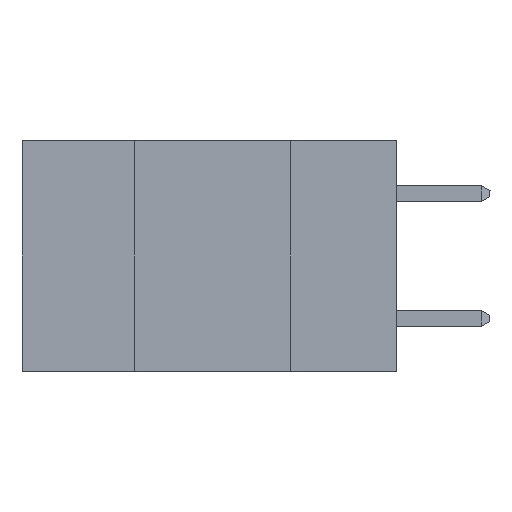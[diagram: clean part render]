
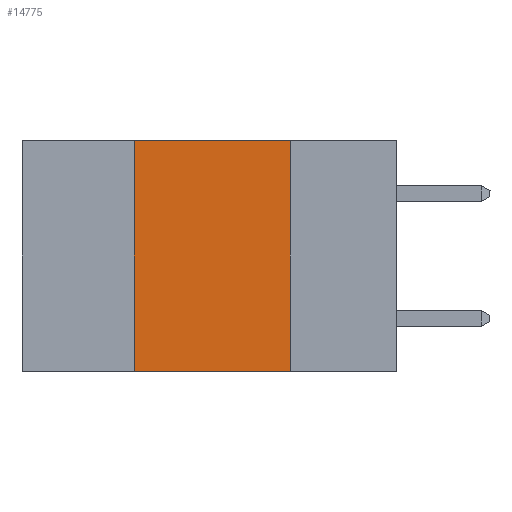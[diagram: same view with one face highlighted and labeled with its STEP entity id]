
A CAD part, left-side view. The second image highlights one B-rep face of the part: STEP entity #14775.
In plain terms, the highlighted planar face has unit normal (-1, 0, 0).
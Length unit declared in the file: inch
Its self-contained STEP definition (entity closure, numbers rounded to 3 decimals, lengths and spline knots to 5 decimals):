
#66 = CARTESIAN_POINT ( 'NONE',  ( 0., 0.42, 0. ) ) ;
#1553 = EDGE_CURVE ( 'NONE', #14657, #10902, #3819, .T. ) ;
#2326 = DIRECTION ( 'NONE',  ( 0., 0., 1. ) ) ;
#2853 = CARTESIAN_POINT ( 'NONE',  ( 0., 0.17, 0. ) ) ;
#3294 = CARTESIAN_POINT ( 'NONE',  ( 0., 0.17, 0. ) ) ;
#3672 = EDGE_CURVE ( 'NONE', #7648, #10902, #11378, .T. ) ;
#3819 = LINE ( 'NONE', #3294, #26152 ) ;
#4571 = VECTOR ( 'NONE', #2326, 39.37008 ) ;
#6388 = EDGE_LOOP ( 'NONE', ( #7945, #23681, #28286, #14852 ) ) ;
#6788 = DIRECTION ( 'NONE',  ( 0., 0., -1. ) ) ;
#6940 = FACE_OUTER_BOUND ( 'NONE', #6388, .T. ) ;
#7648 = VERTEX_POINT ( 'NONE', #14026 ) ;
#7729 = PLANE ( 'NONE',  #8079 ) ;
#7945 = ORIENTED_EDGE ( 'NONE', *, *, #1553, .F. ) ;
#8079 = AXIS2_PLACEMENT_3D ( 'NONE', #14413, #12248, #27793 ) ;
#8176 = EDGE_CURVE ( 'NONE', #7648, #18241, #10521, .T. ) ;
#9733 = CARTESIAN_POINT ( 'NONE',  ( 0., 0.42, 0. ) ) ;
#10521 = LINE ( 'NONE', #66, #4571 ) ;
#10902 = VERTEX_POINT ( 'NONE', #18026 ) ;
#11378 = LINE ( 'NONE', #26590, #28400 ) ;
#12248 = DIRECTION ( 'NONE',  ( 1., 0., 0. ) ) ;
#13929 = EDGE_CURVE ( 'NONE', #18241, #14657, #23408, .T. ) ;
#14026 = CARTESIAN_POINT ( 'NONE',  ( 0., 0.42, -0.37 ) ) ;
#14413 = CARTESIAN_POINT ( 'NONE',  ( 0., 0.6, 0. ) ) ;
#14657 = VERTEX_POINT ( 'NONE', #2853 ) ;
#14775 = ADVANCED_FACE ( 'NONE', ( #6940 ), #7729, .F. ) ;
#14823 = DIRECTION ( 'NONE',  ( 0., -1., 0. ) ) ;
#14852 = ORIENTED_EDGE ( 'NONE', *, *, #3672, .T. ) ;
#17520 = VECTOR ( 'NONE', #22715, 39.37008 ) ;
#18026 = CARTESIAN_POINT ( 'NONE',  ( 0., 0.17, -0.37 ) ) ;
#18241 = VERTEX_POINT ( 'NONE', #9733 ) ;
#20496 = CARTESIAN_POINT ( 'NONE',  ( 0., 0.6, 0. ) ) ;
#22715 = DIRECTION ( 'NONE',  ( 0., -1., 0. ) ) ;
#23408 = LINE ( 'NONE', #20496, #17520 ) ;
#23681 = ORIENTED_EDGE ( 'NONE', *, *, #13929, .F. ) ;
#26152 = VECTOR ( 'NONE', #6788, 39.37008 ) ;
#26590 = CARTESIAN_POINT ( 'NONE',  ( 0., 0.6, -0.37 ) ) ;
#27793 = DIRECTION ( 'NONE',  ( 0., 0., -1. ) ) ;
#28286 = ORIENTED_EDGE ( 'NONE', *, *, #8176, .F. ) ;
#28400 = VECTOR ( 'NONE', #14823, 39.37008 ) ;
